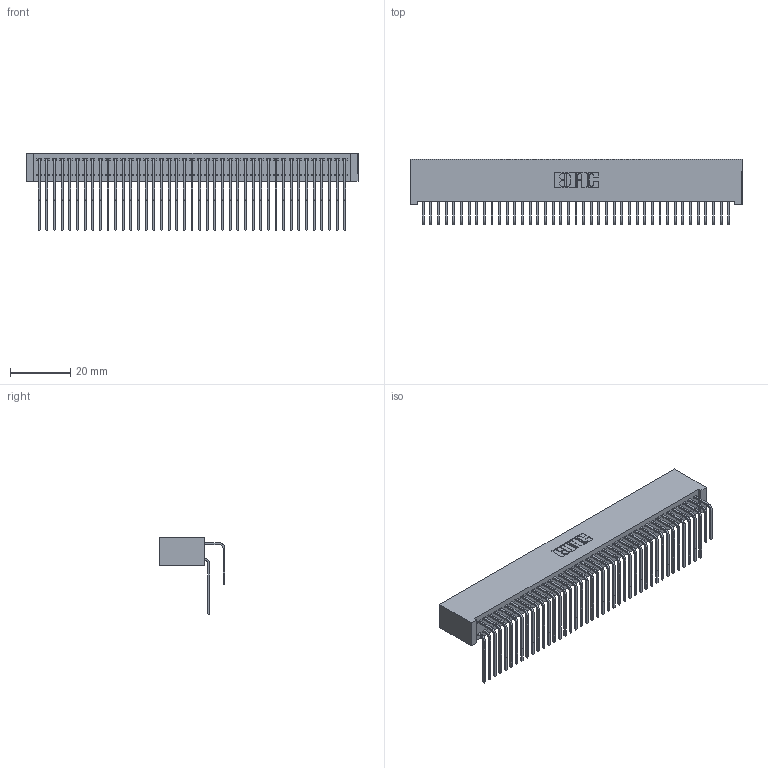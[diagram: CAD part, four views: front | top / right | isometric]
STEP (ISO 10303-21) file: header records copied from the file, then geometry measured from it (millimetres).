
FILE_DESCRIPTION (( 'STEP AP203' ), '1' );
FILE_NAME ('392-082-558-201.STEP', '2019-10-09T15:17:23', ( '' ), ( '' ), 'SwSTEP 2.0', 'SolidWorks 2016', '' );
FILE_SCHEMA (( 'CONFIG_CONTROL_DESIGN' ));
Length unit declared in the file: inch
Products named in the file (4): 345-292-001_558 Tail - 2; 392-082-558-201; 342 Part_Lugless; 345-292-001_558 559 Tail - 1
Assembly tree (83 placements, depth 2):
  392-082-558-201
    342 Part_Lugless
    345-292-001_558 559 Tail - 1  x41
    345-292-001_558 Tail - 2  x41
Bounding box: 110.39 x 21.91 x 25.78 mm (x, y, z)
Volume: 10826.2 mm3; surface area: 20183.8 mm2
Topology: 83 solids, 83 shells, 4530 faces, 13477 edges, 8874 vertices
Faces by surface type: plane 3178, cylinder 1352
Entity records: 27881 total; most frequent: CARTESIAN_POINT 4669, ORIENTED_EDGE 4554, DIRECTION 3965, EDGE_CURVE 2277, LINE 2117, VECTOR 2117, VERTEX_POINT 1514, AXIS2_PLACEMENT_3D 924
